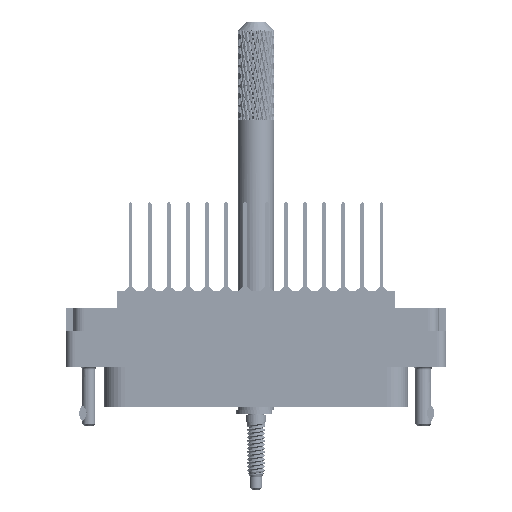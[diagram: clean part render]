
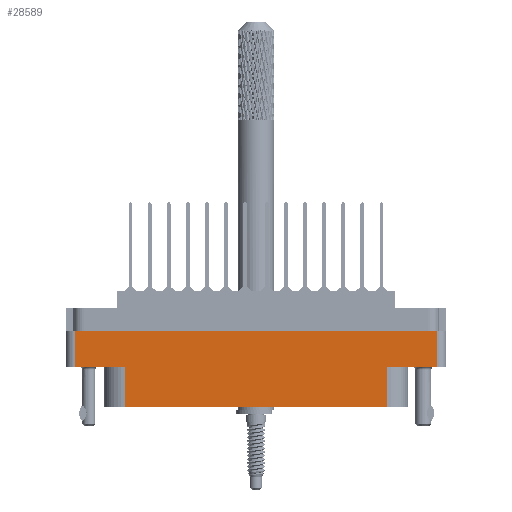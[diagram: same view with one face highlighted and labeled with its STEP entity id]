
A CAD part, front view. The second image highlights one B-rep face of the part: STEP entity #28589.
In plain terms, the highlighted planar face has unit normal (0, -1, 0).
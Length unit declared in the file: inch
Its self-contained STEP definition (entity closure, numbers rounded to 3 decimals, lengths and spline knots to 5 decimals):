
#455 = ORIENTED_EDGE ( 'NONE', *, *, #59946, .F. ) ;
#538 = CARTESIAN_POINT ( 'NONE',  ( 0., -0.438, -0.274 ) ) ;
#3764 = DIRECTION ( 'NONE',  ( 0., 0., 1. ) ) ;
#6682 = ORIENTED_EDGE ( 'NONE', *, *, #50548, .T. ) ;
#6832 = CARTESIAN_POINT ( 'NONE',  ( -1.2335, -0.438, -0.789 ) ) ;
#7176 = VERTEX_POINT ( 'NONE', #69903 ) ;
#11467 = VECTOR ( 'NONE', #120178, 39.37008 ) ;
#17913 = VERTEX_POINT ( 'NONE', #55167 ) ;
#18339 = CARTESIAN_POINT ( 'NONE',  ( -0.895, -0.438, -0.52 ) ) ;
#18878 = VERTEX_POINT ( 'NONE', #92011 ) ;
#21647 = LINE ( 'NONE', #109934, #75711 ) ;
#27914 = ORIENTED_EDGE ( 'NONE', *, *, #30941, .F. ) ;
#28589 = ADVANCED_FACE ( 'NONE', ( #100493 ), #74243, .T. ) ;
#29862 = LINE ( 'NONE', #538, #79030 ) ;
#30941 = EDGE_CURVE ( 'NONE', #83253, #74439, #29862, .T. ) ;
#33009 = VECTOR ( 'NONE', #37892, 39.37008 ) ;
#33074 = ORIENTED_EDGE ( 'NONE', *, *, #116112, .T. ) ;
#33770 = ORIENTED_EDGE ( 'NONE', *, *, #108751, .T. ) ;
#34472 = LINE ( 'NONE', #109669, #40509 ) ;
#34910 = CARTESIAN_POINT ( 'NONE',  ( 0., -0.438, -0.52 ) ) ;
#35544 = CARTESIAN_POINT ( 'NONE',  ( 1.2335, -0.438, -0.274 ) ) ;
#37852 = LINE ( 'NONE', #41567, #91971 ) ;
#37892 = DIRECTION ( 'NONE',  ( 0., 0., -1. ) ) ;
#39013 = DIRECTION ( 'NONE',  ( 0., 0., -1. ) ) ;
#39497 = ORIENTED_EDGE ( 'NONE', *, *, #62134, .F. ) ;
#40509 = VECTOR ( 'NONE', #90388, 39.37008 ) ;
#41567 = CARTESIAN_POINT ( 'NONE',  ( 0.895, -0.438, -0.52 ) ) ;
#44958 = DIRECTION ( 'NONE',  ( -1., 0., 0. ) ) ;
#45056 = LINE ( 'NONE', #6832, #33009 ) ;
#48574 = CARTESIAN_POINT ( 'NONE',  ( -1.2955, -0.438, -0.789 ) ) ;
#50548 = EDGE_CURVE ( 'NONE', #80423, #18878, #55208, .T. ) ;
#52349 = DIRECTION ( 'NONE',  ( -1., 0., 0. ) ) ;
#52368 = CARTESIAN_POINT ( 'NONE',  ( -1.2955, -0.438, -0.789 ) ) ;
#55167 = CARTESIAN_POINT ( 'NONE',  ( 0.895, -0.438, -0.52 ) ) ;
#55208 = LINE ( 'NONE', #52368, #88353 ) ;
#56040 = CARTESIAN_POINT ( 'NONE',  ( -1.2335, -0.438, -0.274 ) ) ;
#59946 = EDGE_CURVE ( 'NONE', #7176, #17913, #21647, .T. ) ;
#62039 = ORIENTED_EDGE ( 'NONE', *, *, #75062, .T. ) ;
#62134 = EDGE_CURVE ( 'NONE', #62654, #102719, #120639, .T. ) ;
#62528 = CARTESIAN_POINT ( 'NONE',  ( -0.895, -0.438, -0.789 ) ) ;
#62654 = VERTEX_POINT ( 'NONE', #18339 ) ;
#67611 = DIRECTION ( 'NONE',  ( 1., 0., 0. ) ) ;
#69903 = CARTESIAN_POINT ( 'NONE',  ( 1.2335, -0.438, -0.52 ) ) ;
#69931 = LINE ( 'NONE', #62528, #11467 ) ;
#70460 = CARTESIAN_POINT ( 'NONE',  ( -0.895, -0.438, -0.789 ) ) ;
#73730 = AXIS2_PLACEMENT_3D ( 'NONE', #48574, #116256, #39013 ) ;
#74243 = PLANE ( 'NONE',  #73730 ) ;
#74439 = VERTEX_POINT ( 'NONE', #35544 ) ;
#75062 = EDGE_CURVE ( 'NONE', #83253, #102719, #45056, .T. ) ;
#75526 = VECTOR ( 'NONE', #44958, 39.37008 ) ;
#75711 = VECTOR ( 'NONE', #52349, 39.37008 ) ;
#79030 = VECTOR ( 'NONE', #67611, 39.37008 ) ;
#80423 = VERTEX_POINT ( 'NONE', #70460 ) ;
#81380 = DIRECTION ( 'NONE',  ( 1., 0., 0. ) ) ;
#83253 = VERTEX_POINT ( 'NONE', #56040 ) ;
#88353 = VECTOR ( 'NONE', #81380, 39.37008 ) ;
#89417 = CARTESIAN_POINT ( 'NONE',  ( -1.2335, -0.438, -0.52 ) ) ;
#90388 = DIRECTION ( 'NONE',  ( 0., 0., 1. ) ) ;
#91971 = VECTOR ( 'NONE', #3764, 39.37008 ) ;
#92011 = CARTESIAN_POINT ( 'NONE',  ( 0.895, -0.438, -0.789 ) ) ;
#100493 = FACE_OUTER_BOUND ( 'NONE', #104852, .T. ) ;
#100704 = ORIENTED_EDGE ( 'NONE', *, *, #112654, .T. ) ;
#102719 = VERTEX_POINT ( 'NONE', #89417 ) ;
#104852 = EDGE_LOOP ( 'NONE', ( #27914, #62039, #39497, #33074, #6682, #33770, #455, #100704 ) ) ;
#108751 = EDGE_CURVE ( 'NONE', #18878, #17913, #37852, .T. ) ;
#109669 = CARTESIAN_POINT ( 'NONE',  ( 1.2335, -0.438, -0.789 ) ) ;
#109934 = CARTESIAN_POINT ( 'NONE',  ( 0., -0.438, -0.52 ) ) ;
#112654 = EDGE_CURVE ( 'NONE', #7176, #74439, #34472, .T. ) ;
#116112 = EDGE_CURVE ( 'NONE', #62654, #80423, #69931, .T. ) ;
#116256 = DIRECTION ( 'NONE',  ( 0., -1., 0. ) ) ;
#120178 = DIRECTION ( 'NONE',  ( 0., 0., -1. ) ) ;
#120639 = LINE ( 'NONE', #34910, #75526 ) ;
